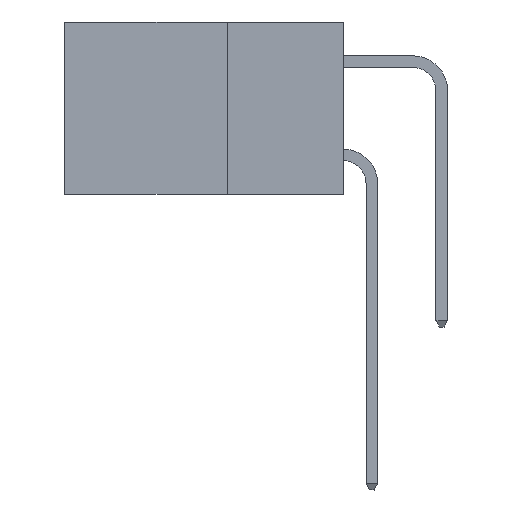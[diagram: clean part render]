
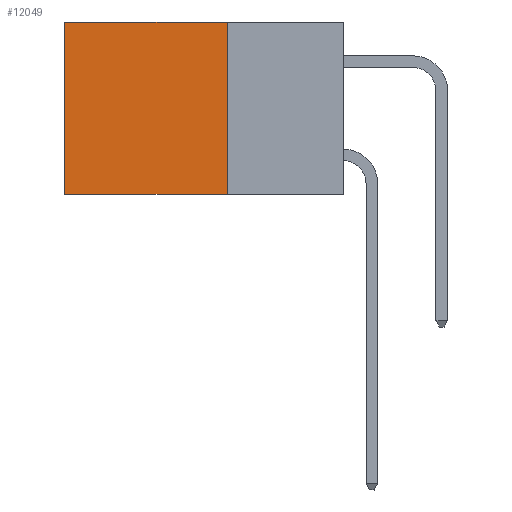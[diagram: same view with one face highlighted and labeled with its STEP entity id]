
A CAD part, left-side view. The second image highlights one B-rep face of the part: STEP entity #12049.
In plain terms, the highlighted planar face has unit normal (-1, 0, 0).
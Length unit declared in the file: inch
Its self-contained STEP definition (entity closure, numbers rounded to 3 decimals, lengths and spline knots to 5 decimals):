
#1416 = DIRECTION ( 'NONE',  ( 0., 0., -1. ) ) ;
#2257 = LINE ( 'NONE', #16489, #20884 ) ;
#2283 = VERTEX_POINT ( 'NONE', #6056 ) ;
#2625 = PLANE ( 'NONE',  #5636 ) ;
#2948 = CARTESIAN_POINT ( 'NONE',  ( 0.298, 0.25, -0.37 ) ) ;
#3031 = VECTOR ( 'NONE', #7201, 39.37008 ) ;
#4278 = EDGE_LOOP ( 'NONE', ( #4541, #20335, #9437, #19400 ) ) ;
#4505 = DIRECTION ( 'NONE',  ( 0., 0., -1. ) ) ;
#4541 = ORIENTED_EDGE ( 'NONE', *, *, #19212, .T. ) ;
#4627 = EDGE_CURVE ( 'NONE', #12480, #9879, #8200, .T. ) ;
#5636 = AXIS2_PLACEMENT_3D ( 'NONE', #22417, #15281, #4505 ) ;
#6036 = FACE_OUTER_BOUND ( 'NONE', #4278, .T. ) ;
#6056 = CARTESIAN_POINT ( 'NONE',  ( 0.298, 0.6, 0. ) ) ;
#7201 = DIRECTION ( 'NONE',  ( 0., 0., -1. ) ) ;
#8200 = LINE ( 'NONE', #11814, #21884 ) ;
#9437 = ORIENTED_EDGE ( 'NONE', *, *, #4627, .F. ) ;
#9879 = VERTEX_POINT ( 'NONE', #2948 ) ;
#10497 = EDGE_CURVE ( 'NONE', #9879, #11029, #16497, .T. ) ;
#11029 = VERTEX_POINT ( 'NONE', #16938 ) ;
#11814 = CARTESIAN_POINT ( 'NONE',  ( 0.298, 0.25, 0. ) ) ;
#12049 = ADVANCED_FACE ( 'NONE', ( #6036 ), #2625, .F. ) ;
#12480 = VERTEX_POINT ( 'NONE', #20029 ) ;
#15281 = DIRECTION ( 'NONE',  ( 1., 0., 0. ) ) ;
#15337 = DIRECTION ( 'NONE',  ( 0., 1., 0. ) ) ;
#15933 = VECTOR ( 'NONE', #15337, 39.37008 ) ;
#16489 = CARTESIAN_POINT ( 'NONE',  ( 0.298, 0.25, 0. ) ) ;
#16497 = LINE ( 'NONE', #17118, #15933 ) ;
#16938 = CARTESIAN_POINT ( 'NONE',  ( 0.298, 0.6, -0.37 ) ) ;
#17118 = CARTESIAN_POINT ( 'NONE',  ( 0.298, 0.25, -0.37 ) ) ;
#18280 = DIRECTION ( 'NONE',  ( 0., 1., 0. ) ) ;
#19212 = EDGE_CURVE ( 'NONE', #2283, #11029, #21632, .T. ) ;
#19400 = ORIENTED_EDGE ( 'NONE', *, *, #22648, .T. ) ;
#19687 = CARTESIAN_POINT ( 'NONE',  ( 0.298, 0.6, 0. ) ) ;
#20029 = CARTESIAN_POINT ( 'NONE',  ( 0.298, 0.25, 0. ) ) ;
#20335 = ORIENTED_EDGE ( 'NONE', *, *, #10497, .F. ) ;
#20884 = VECTOR ( 'NONE', #18280, 39.37008 ) ;
#21632 = LINE ( 'NONE', #19687, #3031 ) ;
#21884 = VECTOR ( 'NONE', #1416, 39.37008 ) ;
#22417 = CARTESIAN_POINT ( 'NONE',  ( 0.298, 0.25, 0. ) ) ;
#22648 = EDGE_CURVE ( 'NONE', #12480, #2283, #2257, .T. ) ;
